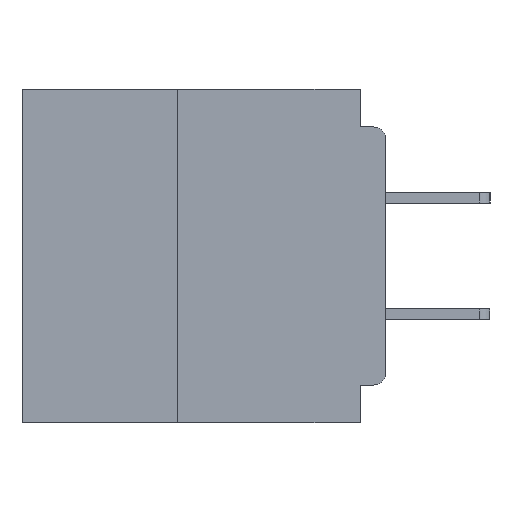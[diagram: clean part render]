
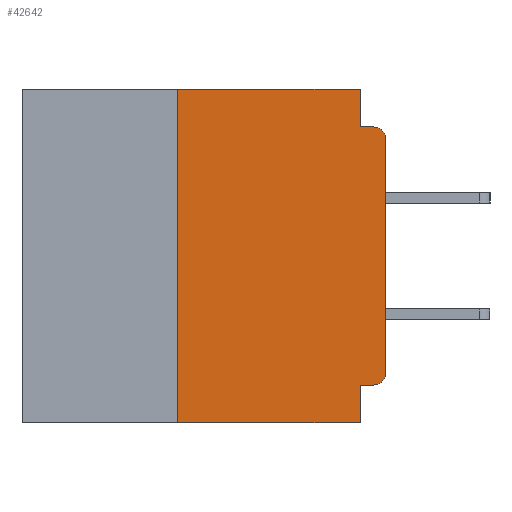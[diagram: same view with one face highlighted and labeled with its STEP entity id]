
A CAD part, left-side view. The second image highlights one B-rep face of the part: STEP entity #42642.
In plain terms, the highlighted planar face has unit normal (-1, 0, 0).
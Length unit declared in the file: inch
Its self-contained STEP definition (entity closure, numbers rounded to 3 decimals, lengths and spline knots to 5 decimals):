
#1532 = CARTESIAN_POINT ( 'NONE',  ( 0., 0.015, -0.355 ) ) ;
#1575 = AXIS2_PLACEMENT_3D ( 'NONE', #47786, #21310, #52192 ) ;
#1932 = ORIENTED_EDGE ( 'NONE', *, *, #7831, .T. ) ;
#3800 = VECTOR ( 'NONE', #37297, 39.37008 ) ;
#3986 = EDGE_CURVE ( 'NONE', #22168, #11665, #12363, .T. ) ;
#4119 = ORIENTED_EDGE ( 'NONE', *, *, #21305, .F. ) ;
#5410 = CIRCLE ( 'NONE', #14099, 0.015 ) ;
#5721 = VERTEX_POINT ( 'NONE', #38350 ) ;
#6755 = VERTEX_POINT ( 'NONE', #19325 ) ;
#7251 = EDGE_CURVE ( 'NONE', #11665, #25836, #34760, .T. ) ;
#7831 = EDGE_CURVE ( 'NONE', #49509, #5721, #51302, .T. ) ;
#8357 = VERTEX_POINT ( 'NONE', #38042 ) ;
#10196 = LINE ( 'NONE', #10327, #22046 ) ;
#10289 = DIRECTION ( 'NONE',  ( 0., 0., -1. ) ) ;
#10327 = CARTESIAN_POINT ( 'NONE',  ( 0., 0.437, -0.4 ) ) ;
#11665 = VERTEX_POINT ( 'NONE', #50783 ) ;
#12310 = VERTEX_POINT ( 'NONE', #55347 ) ;
#12363 = LINE ( 'NONE', #39206, #24182 ) ;
#12810 = CARTESIAN_POINT ( 'NONE',  ( 0., 0.031, -0.4 ) ) ;
#12868 = DIRECTION ( 'NONE',  ( -1., 0., 0. ) ) ;
#14011 = CARTESIAN_POINT ( 'NONE',  ( 0., 0.031, 0. ) ) ;
#14099 = AXIS2_PLACEMENT_3D ( 'NONE', #39365, #12868, #43837 ) ;
#14847 = LINE ( 'NONE', #45683, #28007 ) ;
#16078 = VERTEX_POINT ( 'NONE', #43127 ) ;
#17336 = AXIS2_PLACEMENT_3D ( 'NONE', #19232, #36798, #28113 ) ;
#17908 = CARTESIAN_POINT ( 'NONE',  ( 0., 0.015, -0.045 ) ) ;
#17937 = VERTEX_POINT ( 'NONE', #17908 ) ;
#18122 = CARTESIAN_POINT ( 'NONE',  ( 0., 0.437, 0. ) ) ;
#18673 = VECTOR ( 'NONE', #43782, 39.37008 ) ;
#19232 = CARTESIAN_POINT ( 'NONE',  ( 0., 0.437, 0. ) ) ;
#19325 = CARTESIAN_POINT ( 'NONE',  ( 0., 0.031, -0.4 ) ) ;
#20021 = EDGE_CURVE ( 'NONE', #12310, #6755, #55263, .T. ) ;
#21305 = EDGE_CURVE ( 'NONE', #16078, #17937, #53018, .T. ) ;
#21310 = DIRECTION ( 'NONE',  ( -1., 0., 0. ) ) ;
#21805 = ORIENTED_EDGE ( 'NONE', *, *, #20021, .F. ) ;
#22046 = VECTOR ( 'NONE', #41322, 39.37008 ) ;
#22168 = VERTEX_POINT ( 'NONE', #25186 ) ;
#22998 = ORIENTED_EDGE ( 'NONE', *, *, #56790, .T. ) ;
#23091 = VECTOR ( 'NONE', #31389, 39.37008 ) ;
#23490 = DIRECTION ( 'NONE',  ( 0., 1., 0. ) ) ;
#23711 = PLANE ( 'NONE',  #17336 ) ;
#24182 = VECTOR ( 'NONE', #39340, 39.37008 ) ;
#25186 = CARTESIAN_POINT ( 'NONE',  ( 0., 0.25, -0.4 ) ) ;
#25420 = ORIENTED_EDGE ( 'NONE', *, *, #25704, .T. ) ;
#25704 = EDGE_CURVE ( 'NONE', #8357, #17937, #5410, .T. ) ;
#25836 = VERTEX_POINT ( 'NONE', #14011 ) ;
#27788 = EDGE_CURVE ( 'NONE', #25836, #16078, #29844, .T. ) ;
#28007 = VECTOR ( 'NONE', #23490, 39.37008 ) ;
#28083 = ORIENTED_EDGE ( 'NONE', *, *, #27788, .F. ) ;
#28113 = DIRECTION ( 'NONE',  ( 0., 0., -1. ) ) ;
#28783 = LINE ( 'NONE', #46014, #3800 ) ;
#29844 = LINE ( 'NONE', #41298, #54723 ) ;
#31389 = DIRECTION ( 'NONE',  ( 0., -1., 0. ) ) ;
#34760 = LINE ( 'NONE', #18122, #23091 ) ;
#35415 = ORIENTED_EDGE ( 'NONE', *, *, #3986, .F. ) ;
#36593 = FACE_OUTER_BOUND ( 'NONE', #55198, .T. ) ;
#36798 = DIRECTION ( 'NONE',  ( 1., 0., 0. ) ) ;
#37297 = DIRECTION ( 'NONE',  ( 0., 0., 1. ) ) ;
#38042 = CARTESIAN_POINT ( 'NONE',  ( 0., 0., -0.06 ) ) ;
#38350 = CARTESIAN_POINT ( 'NONE',  ( 0., 0., -0.34 ) ) ;
#39169 = CARTESIAN_POINT ( 'NONE',  ( 0., 0., -0.045 ) ) ;
#39206 = CARTESIAN_POINT ( 'NONE',  ( 0., 0.25, -0.4 ) ) ;
#39216 = ORIENTED_EDGE ( 'NONE', *, *, #55505, .T. ) ;
#39340 = DIRECTION ( 'NONE',  ( 0., 0., 1. ) ) ;
#39365 = CARTESIAN_POINT ( 'NONE',  ( 0., 0.015, -0.06 ) ) ;
#40379 = ORIENTED_EDGE ( 'NONE', *, *, #46415, .F. ) ;
#41298 = CARTESIAN_POINT ( 'NONE',  ( 0., 0.031, 0. ) ) ;
#41322 = DIRECTION ( 'NONE',  ( 0., -1., 0. ) ) ;
#42642 = ADVANCED_FACE ( 'NONE', ( #36593 ), #23711, .F. ) ;
#43127 = CARTESIAN_POINT ( 'NONE',  ( 0., 0.031, -0.045 ) ) ;
#43782 = DIRECTION ( 'NONE',  ( 0., 0., -1. ) ) ;
#43837 = DIRECTION ( 'NONE',  ( 0., 0., -1. ) ) ;
#45683 = CARTESIAN_POINT ( 'NONE',  ( 0., 0., -0.355 ) ) ;
#46014 = CARTESIAN_POINT ( 'NONE',  ( 0., 0., 0. ) ) ;
#46415 = EDGE_CURVE ( 'NONE', #49509, #12310, #14847, .T. ) ;
#47786 = CARTESIAN_POINT ( 'NONE',  ( 0., 0.015, -0.34 ) ) ;
#49509 = VERTEX_POINT ( 'NONE', #1532 ) ;
#50783 = CARTESIAN_POINT ( 'NONE',  ( 0., 0.25, 0. ) ) ;
#51302 = CIRCLE ( 'NONE', #1575, 0.015 ) ;
#51624 = VECTOR ( 'NONE', #56899, 39.37008 ) ;
#52192 = DIRECTION ( 'NONE',  ( 0., 0., -1. ) ) ;
#53018 = LINE ( 'NONE', #39169, #51624 ) ;
#54723 = VECTOR ( 'NONE', #10289, 39.37008 ) ;
#55198 = EDGE_LOOP ( 'NONE', ( #22998, #25420, #4119, #28083, #56849, #35415, #39216, #21805, #40379, #1932 ) ) ;
#55263 = LINE ( 'NONE', #12810, #18673 ) ;
#55347 = CARTESIAN_POINT ( 'NONE',  ( 0., 0.031, -0.355 ) ) ;
#55505 = EDGE_CURVE ( 'NONE', #22168, #6755, #10196, .T. ) ;
#56790 = EDGE_CURVE ( 'NONE', #5721, #8357, #28783, .T. ) ;
#56849 = ORIENTED_EDGE ( 'NONE', *, *, #7251, .F. ) ;
#56899 = DIRECTION ( 'NONE',  ( 0., -1., 0. ) ) ;
